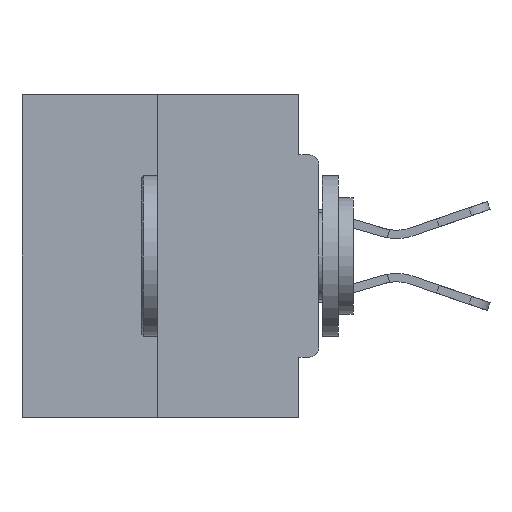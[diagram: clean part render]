
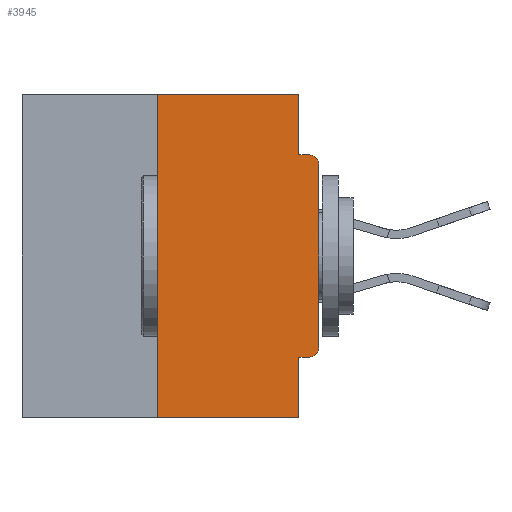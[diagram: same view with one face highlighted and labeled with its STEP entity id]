
A CAD part, left-side view. The second image highlights one B-rep face of the part: STEP entity #3945.
In plain terms, the highlighted planar face has unit normal (-1, 0, 0).
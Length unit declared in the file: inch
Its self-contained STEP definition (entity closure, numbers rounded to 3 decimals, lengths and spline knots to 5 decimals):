
#150 = CARTESIAN_POINT ( 'NONE',  ( 0., 0.015, -0.4065 ) ) ;
#416 = CARTESIAN_POINT ( 'NONE',  ( 0., 0.015, -0.1085 ) ) ;
#1014 = VERTEX_POINT ( 'NONE', #14760 ) ;
#1668 = VECTOR ( 'NONE', #38071, 39.37008 ) ;
#2459 = LINE ( 'NONE', #10163, #36960 ) ;
#2473 = EDGE_CURVE ( 'NONE', #1014, #34086, #3882, .T. ) ;
#2863 = LINE ( 'NONE', #25233, #35758 ) ;
#3882 = LINE ( 'NONE', #13638, #42025 ) ;
#3945 = ADVANCED_FACE ( 'NONE', ( #29383 ), #12463, .F. ) ;
#5214 = CARTESIAN_POINT ( 'NONE',  ( 0., 0.031, -0.4065 ) ) ;
#5429 = DIRECTION ( 'NONE',  ( 0., 0., -1. ) ) ;
#5728 = CARTESIAN_POINT ( 'NONE',  ( 0., 0.46, 0. ) ) ;
#5844 = CARTESIAN_POINT ( 'NONE',  ( 0., 0.46, -0.5 ) ) ;
#6369 = EDGE_CURVE ( 'NONE', #38614, #25773, #26525, .T. ) ;
#6874 = ORIENTED_EDGE ( 'NONE', *, *, #7909, .F. ) ;
#7023 = CARTESIAN_POINT ( 'NONE',  ( 0., 0.25, 0. ) ) ;
#7039 = EDGE_CURVE ( 'NONE', #31630, #20239, #17982, .T. ) ;
#7096 = ORIENTED_EDGE ( 'NONE', *, *, #8804, .F. ) ;
#7491 = DIRECTION ( 'NONE',  ( 0., 1., 0. ) ) ;
#7909 = EDGE_CURVE ( 'NONE', #34138, #35756, #40425, .T. ) ;
#7983 = CARTESIAN_POINT ( 'NONE',  ( 0., 0.015, -0.0935 ) ) ;
#8804 = EDGE_CURVE ( 'NONE', #20239, #19000, #24168, .T. ) ;
#9202 = DIRECTION ( 'NONE',  ( 0., -1., 0. ) ) ;
#9620 = EDGE_CURVE ( 'NONE', #38614, #34138, #15228, .T. ) ;
#10163 = CARTESIAN_POINT ( 'NONE',  ( 0., 0.031, 0. ) ) ;
#10777 = CARTESIAN_POINT ( 'NONE',  ( 0., 0.015, -0.3915 ) ) ;
#10899 = CARTESIAN_POINT ( 'NONE',  ( 0., 0.25, -0.5 ) ) ;
#11614 = ORIENTED_EDGE ( 'NONE', *, *, #2473, .F. ) ;
#11770 = EDGE_CURVE ( 'NONE', #19000, #1014, #2459, .T. ) ;
#11902 = CARTESIAN_POINT ( 'NONE',  ( 0., 0.031, -0.5 ) ) ;
#11984 = AXIS2_PLACEMENT_3D ( 'NONE', #416, #23419, #43262 ) ;
#12036 = DIRECTION ( 'NONE',  ( 1., 0., 0. ) ) ;
#12125 = VECTOR ( 'NONE', #7491, 39.37008 ) ;
#12463 = PLANE ( 'NONE',  #43272 ) ;
#13258 = DIRECTION ( 'NONE',  ( 0., 0., -1. ) ) ;
#13271 = ORIENTED_EDGE ( 'NONE', *, *, #34350, .T. ) ;
#13638 = CARTESIAN_POINT ( 'NONE',  ( 0., 0., -0.0935 ) ) ;
#14282 = DIRECTION ( 'NONE',  ( -1., 0., 0. ) ) ;
#14760 = CARTESIAN_POINT ( 'NONE',  ( 0., 0.031, -0.0935 ) ) ;
#15228 = LINE ( 'NONE', #27924, #12125 ) ;
#15414 = EDGE_LOOP ( 'NONE', ( #7096, #23147, #37378, #6874, #26358, #37841, #40489, #13271, #11614, #17000 ) ) ;
#16938 = DIRECTION ( 'NONE',  ( 0., -1., 0. ) ) ;
#17000 = ORIENTED_EDGE ( 'NONE', *, *, #11770, .F. ) ;
#17982 = LINE ( 'NONE', #7023, #22739 ) ;
#19000 = VERTEX_POINT ( 'NONE', #41235 ) ;
#20239 = VERTEX_POINT ( 'NONE', #35279 ) ;
#20255 = DIRECTION ( 'NONE',  ( 0., 0., -1. ) ) ;
#20440 = DIRECTION ( 'NONE',  ( 0., 0., 1. ) ) ;
#21849 = DIRECTION ( 'NONE',  ( 0., 0., -1. ) ) ;
#22739 = VECTOR ( 'NONE', #20440, 39.37008 ) ;
#23147 = ORIENTED_EDGE ( 'NONE', *, *, #7039, .F. ) ;
#23419 = DIRECTION ( 'NONE',  ( -1., 0., 0. ) ) ;
#24168 = LINE ( 'NONE', #41325, #1668 ) ;
#25233 = CARTESIAN_POINT ( 'NONE',  ( 0., 0., 0. ) ) ;
#25496 = CARTESIAN_POINT ( 'NONE',  ( 0., 0.031, -0.5 ) ) ;
#25773 = VERTEX_POINT ( 'NONE', #26879 ) ;
#26358 = ORIENTED_EDGE ( 'NONE', *, *, #9620, .F. ) ;
#26525 = CIRCLE ( 'NONE', #41678, 0.015 ) ;
#26879 = CARTESIAN_POINT ( 'NONE',  ( 0., 0., -0.3915 ) ) ;
#27924 = CARTESIAN_POINT ( 'NONE',  ( 0., 0., -0.4065 ) ) ;
#28031 = DIRECTION ( 'NONE',  ( 0., 0., 1. ) ) ;
#29383 = FACE_OUTER_BOUND ( 'NONE', #15414, .T. ) ;
#31129 = VERTEX_POINT ( 'NONE', #38623 ) ;
#31630 = VERTEX_POINT ( 'NONE', #10899 ) ;
#33909 = EDGE_CURVE ( 'NONE', #31630, #35756, #37542, .T. ) ;
#34086 = VERTEX_POINT ( 'NONE', #7983 ) ;
#34138 = VERTEX_POINT ( 'NONE', #5214 ) ;
#34350 = EDGE_CURVE ( 'NONE', #31129, #34086, #40667, .T. ) ;
#35172 = VECTOR ( 'NONE', #21849, 39.37008 ) ;
#35279 = CARTESIAN_POINT ( 'NONE',  ( 0., 0.25, 0. ) ) ;
#35756 = VERTEX_POINT ( 'NONE', #11902 ) ;
#35758 = VECTOR ( 'NONE', #28031, 39.37008 ) ;
#36960 = VECTOR ( 'NONE', #13258, 39.37008 ) ;
#37378 = ORIENTED_EDGE ( 'NONE', *, *, #33909, .T. ) ;
#37542 = LINE ( 'NONE', #5844, #39645 ) ;
#37841 = ORIENTED_EDGE ( 'NONE', *, *, #6369, .T. ) ;
#38071 = DIRECTION ( 'NONE',  ( 0., -1., 0. ) ) ;
#38614 = VERTEX_POINT ( 'NONE', #150 ) ;
#38623 = CARTESIAN_POINT ( 'NONE',  ( 0., 0., -0.1085 ) ) ;
#39293 = EDGE_CURVE ( 'NONE', #25773, #31129, #2863, .T. ) ;
#39645 = VECTOR ( 'NONE', #9202, 39.37008 ) ;
#40425 = LINE ( 'NONE', #25496, #35172 ) ;
#40489 = ORIENTED_EDGE ( 'NONE', *, *, #39293, .T. ) ;
#40667 = CIRCLE ( 'NONE', #11984, 0.015 ) ;
#41235 = CARTESIAN_POINT ( 'NONE',  ( 0., 0.031, 0. ) ) ;
#41325 = CARTESIAN_POINT ( 'NONE',  ( 0., 0.46, 0. ) ) ;
#41678 = AXIS2_PLACEMENT_3D ( 'NONE', #10777, #14282, #20255 ) ;
#42025 = VECTOR ( 'NONE', #16938, 39.37008 ) ;
#43262 = DIRECTION ( 'NONE',  ( 0., 0., -1. ) ) ;
#43272 = AXIS2_PLACEMENT_3D ( 'NONE', #5728, #12036, #5429 ) ;
